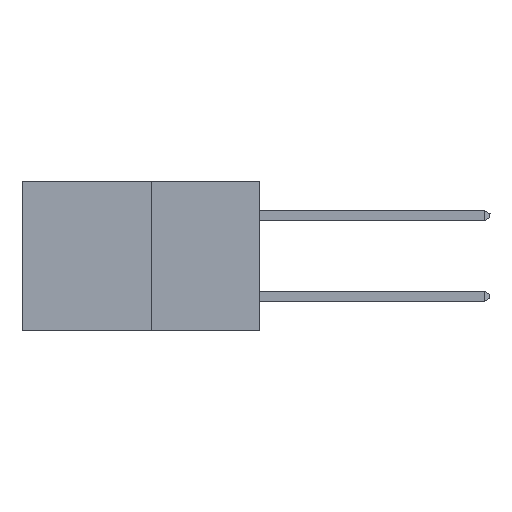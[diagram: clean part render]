
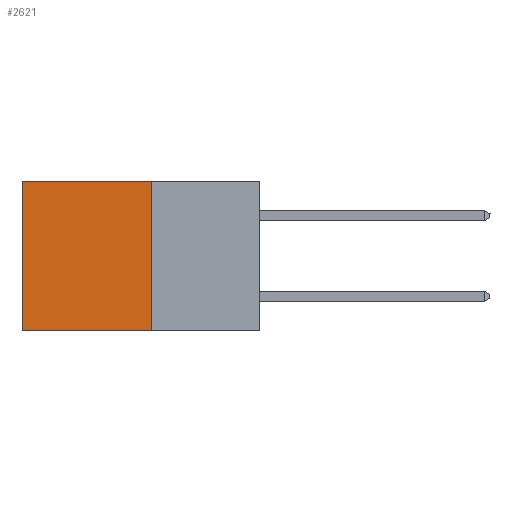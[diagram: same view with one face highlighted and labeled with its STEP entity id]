
A CAD part, left-side view. The second image highlights one B-rep face of the part: STEP entity #2621.
In plain terms, the highlighted planar face has unit normal (-1, 0, 0).
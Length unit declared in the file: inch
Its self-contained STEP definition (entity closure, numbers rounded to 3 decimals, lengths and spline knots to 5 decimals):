
#430 = LINE ( 'NONE', #8658, #2803 ) ;
#485 = DIRECTION ( 'NONE',  ( 0., 0., -1. ) ) ;
#652 = ORIENTED_EDGE ( 'NONE', *, *, #3861, .T. ) ;
#1599 = ORIENTED_EDGE ( 'NONE', *, *, #4247, .T. ) ;
#1621 = ORIENTED_EDGE ( 'NONE', *, *, #9312, .F. ) ;
#1855 = AXIS2_PLACEMENT_3D ( 'NONE', #8118, #6272, #4326 ) ;
#2064 = VECTOR ( 'NONE', #7437, 39.37008 ) ;
#2409 = DIRECTION ( 'NONE',  ( 0., 1., 0. ) ) ;
#2621 = ADVANCED_FACE ( 'NONE', ( #9295 ), #6564, .F. ) ;
#2629 = CARTESIAN_POINT ( 'NONE',  ( 0.277, 0.27, 0. ) ) ;
#2803 = VECTOR ( 'NONE', #485, 39.37008 ) ;
#3280 = CARTESIAN_POINT ( 'NONE',  ( 0.277, 0.59, 0. ) ) ;
#3861 = EDGE_CURVE ( 'NONE', #11261, #10522, #12611, .T. ) ;
#4026 = LINE ( 'NONE', #7706, #11848 ) ;
#4247 = EDGE_CURVE ( 'NONE', #10147, #11261, #7824, .T. ) ;
#4326 = DIRECTION ( 'NONE',  ( 0., 0., -1. ) ) ;
#5149 = VECTOR ( 'NONE', #2409, 39.37008 ) ;
#5363 = CARTESIAN_POINT ( 'NONE',  ( 0.277, 0.59, -0.37 ) ) ;
#5468 = EDGE_LOOP ( 'NONE', ( #652, #1621, #8388, #1599 ) ) ;
#6272 = DIRECTION ( 'NONE',  ( 1., 0., 0. ) ) ;
#6564 = PLANE ( 'NONE',  #1855 ) ;
#7437 = DIRECTION ( 'NONE',  ( 0., 0., -1. ) ) ;
#7445 = CARTESIAN_POINT ( 'NONE',  ( 0.277, 0.59, -0.37 ) ) ;
#7706 = CARTESIAN_POINT ( 'NONE',  ( 0.277, 0.27, -0.37 ) ) ;
#7824 = LINE ( 'NONE', #2629, #5149 ) ;
#7828 = CARTESIAN_POINT ( 'NONE',  ( 0.277, 0.27, 0. ) ) ;
#7919 = CARTESIAN_POINT ( 'NONE',  ( 0.277, 0.27, -0.37 ) ) ;
#8118 = CARTESIAN_POINT ( 'NONE',  ( 0.277, 0.27, -0.37 ) ) ;
#8388 = ORIENTED_EDGE ( 'NONE', *, *, #12168, .F. ) ;
#8658 = CARTESIAN_POINT ( 'NONE',  ( 0.277, 0.27, -0.37 ) ) ;
#8736 = DIRECTION ( 'NONE',  ( 0., 1., 0. ) ) ;
#9295 = FACE_OUTER_BOUND ( 'NONE', #5468, .T. ) ;
#9312 = EDGE_CURVE ( 'NONE', #10189, #10522, #4026, .T. ) ;
#10147 = VERTEX_POINT ( 'NONE', #7828 ) ;
#10189 = VERTEX_POINT ( 'NONE', #7919 ) ;
#10522 = VERTEX_POINT ( 'NONE', #5363 ) ;
#11261 = VERTEX_POINT ( 'NONE', #3280 ) ;
#11848 = VECTOR ( 'NONE', #8736, 39.37008 ) ;
#12168 = EDGE_CURVE ( 'NONE', #10147, #10189, #430, .T. ) ;
#12611 = LINE ( 'NONE', #7445, #2064 ) ;
